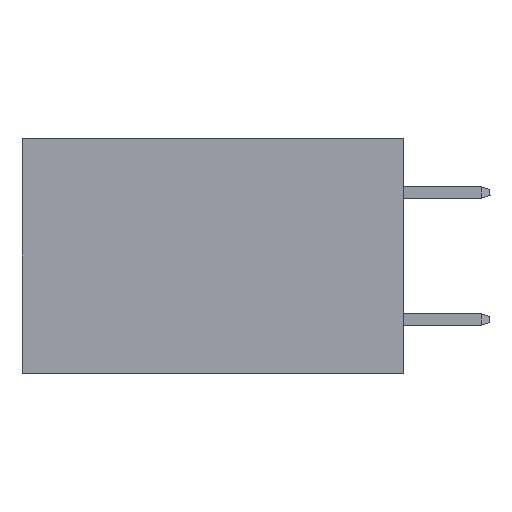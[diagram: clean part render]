
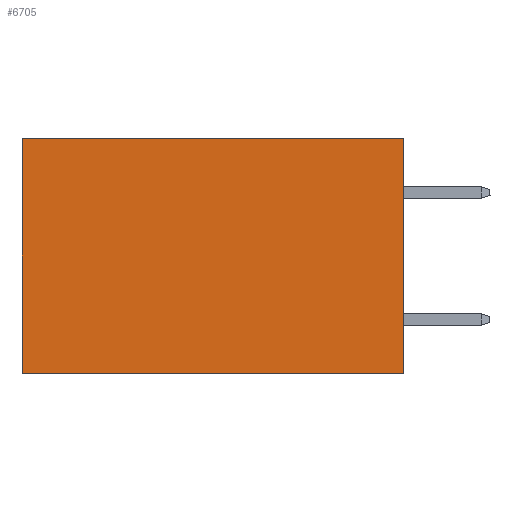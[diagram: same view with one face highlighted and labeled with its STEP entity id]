
A CAD part, left-side view. The second image highlights one B-rep face of the part: STEP entity #6705.
In plain terms, the highlighted planar face has unit normal (-1, 0, 0).
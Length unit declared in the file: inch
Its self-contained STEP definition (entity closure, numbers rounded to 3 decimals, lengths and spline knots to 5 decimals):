
#1199 = DIRECTION ( 'NONE',  ( 0., 1., 0. ) ) ;
#2686 = CARTESIAN_POINT ( 'NONE',  ( 0.2875, 0.6, -0.37 ) ) ;
#4201 = ORIENTED_EDGE ( 'NONE', *, *, #7647, .T. ) ;
#6358 = VECTOR ( 'NONE', #30589, 39.37008 ) ;
#6705 = ADVANCED_FACE ( 'NONE', ( #11472 ), #25622, .F. ) ;
#7647 = EDGE_CURVE ( 'NONE', #11945, #41750, #12731, .T. ) ;
#9910 = VECTOR ( 'NONE', #37900, 39.37008 ) ;
#10238 = VERTEX_POINT ( 'NONE', #33839 ) ;
#11090 = ORIENTED_EDGE ( 'NONE', *, *, #23073, .T. ) ;
#11472 = FACE_OUTER_BOUND ( 'NONE', #45015, .T. ) ;
#11892 = CARTESIAN_POINT ( 'NONE',  ( 0.2875, 0., -0.37 ) ) ;
#11945 = VERTEX_POINT ( 'NONE', #30787 ) ;
#12731 = LINE ( 'NONE', #15511, #39064 ) ;
#15511 = CARTESIAN_POINT ( 'NONE',  ( 0.2875, 0.6, 0. ) ) ;
#15575 = VECTOR ( 'NONE', #1199, 39.37008 ) ;
#16430 = LINE ( 'NONE', #45148, #6358 ) ;
#19732 = VERTEX_POINT ( 'NONE', #30261 ) ;
#19906 = EDGE_CURVE ( 'NONE', #10238, #41750, #32972, .T. ) ;
#20245 = DIRECTION ( 'NONE',  ( 1., 0., 0. ) ) ;
#23073 = EDGE_CURVE ( 'NONE', #19732, #11945, #40906, .T. ) ;
#25622 = PLANE ( 'NONE',  #41952 ) ;
#27248 = CARTESIAN_POINT ( 'NONE',  ( 0.2875, 0., 0. ) ) ;
#30249 = DIRECTION ( 'NONE',  ( 0., 0., -1. ) ) ;
#30261 = CARTESIAN_POINT ( 'NONE',  ( 0.2875, 0., 0. ) ) ;
#30589 = DIRECTION ( 'NONE',  ( 0., 0., -1. ) ) ;
#30787 = CARTESIAN_POINT ( 'NONE',  ( 0.2875, 0.6, 0. ) ) ;
#32972 = LINE ( 'NONE', #11892, #15575 ) ;
#32994 = ORIENTED_EDGE ( 'NONE', *, *, #37262, .F. ) ;
#33839 = CARTESIAN_POINT ( 'NONE',  ( 0.2875, 0., -0.37 ) ) ;
#37262 = EDGE_CURVE ( 'NONE', #19732, #10238, #16430, .T. ) ;
#37854 = CARTESIAN_POINT ( 'NONE',  ( 0.2875, 0., 0. ) ) ;
#37900 = DIRECTION ( 'NONE',  ( 0., 1., 0. ) ) ;
#39064 = VECTOR ( 'NONE', #40529, 39.37008 ) ;
#40529 = DIRECTION ( 'NONE',  ( 0., 0., -1. ) ) ;
#40906 = LINE ( 'NONE', #27248, #9910 ) ;
#41750 = VERTEX_POINT ( 'NONE', #2686 ) ;
#41952 = AXIS2_PLACEMENT_3D ( 'NONE', #37854, #20245, #30249 ) ;
#45015 = EDGE_LOOP ( 'NONE', ( #4201, #45400, #32994, #11090 ) ) ;
#45148 = CARTESIAN_POINT ( 'NONE',  ( 0.2875, 0., 0. ) ) ;
#45400 = ORIENTED_EDGE ( 'NONE', *, *, #19906, .F. ) ;
